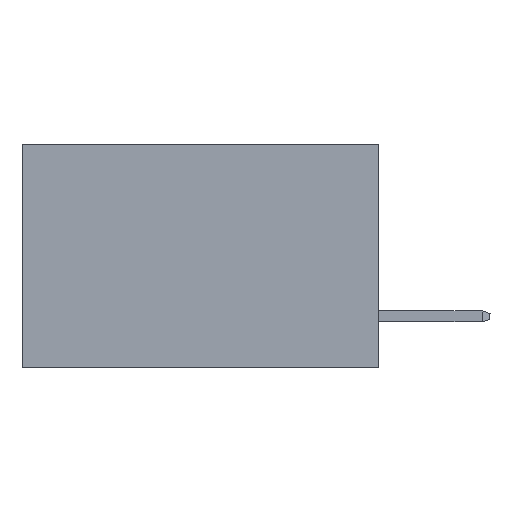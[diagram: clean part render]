
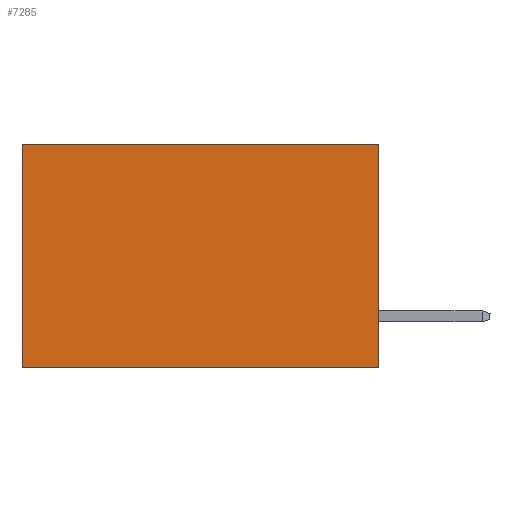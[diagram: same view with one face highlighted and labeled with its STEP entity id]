
A CAD part, left-side view. The second image highlights one B-rep face of the part: STEP entity #7285.
In plain terms, the highlighted planar face has unit normal (-1, 0, 0).
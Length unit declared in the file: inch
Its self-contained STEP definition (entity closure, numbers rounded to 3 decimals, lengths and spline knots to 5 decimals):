
#113 = VERTEX_POINT ( 'NONE', #3536 ) ;
#186 = LINE ( 'NONE', #6970, #7636 ) ;
#222 = CARTESIAN_POINT ( 'NONE',  ( 0.277, 0., -0.37 ) ) ;
#274 = CARTESIAN_POINT ( 'NONE',  ( 0.277, 0., -0.37 ) ) ;
#414 = ORIENTED_EDGE ( 'NONE', *, *, #4793, .F. ) ;
#651 = ORIENTED_EDGE ( 'NONE', *, *, #4095, .F. ) ;
#1653 = VERTEX_POINT ( 'NONE', #2451 ) ;
#1760 = VECTOR ( 'NONE', #8926, 39.37008 ) ;
#1776 = VECTOR ( 'NONE', #3022, 39.37008 ) ;
#1904 = ORIENTED_EDGE ( 'NONE', *, *, #4338, .T. ) ;
#2070 = FACE_OUTER_BOUND ( 'NONE', #3129, .T. ) ;
#2451 = CARTESIAN_POINT ( 'NONE',  ( 0.277, 0.59, 0. ) ) ;
#3022 = DIRECTION ( 'NONE',  ( 0., 0., -1. ) ) ;
#3037 = ORIENTED_EDGE ( 'NONE', *, *, #5791, .T. ) ;
#3129 = EDGE_LOOP ( 'NONE', ( #1904, #414, #651, #3037 ) ) ;
#3536 = CARTESIAN_POINT ( 'NONE',  ( 0.277, 0.59, -0.37 ) ) ;
#3818 = VERTEX_POINT ( 'NONE', #6269 ) ;
#3936 = LINE ( 'NONE', #8883, #1760 ) ;
#4095 = EDGE_CURVE ( 'NONE', #3818, #8555, #186, .T. ) ;
#4338 = EDGE_CURVE ( 'NONE', #1653, #113, #5587, .T. ) ;
#4354 = CARTESIAN_POINT ( 'NONE',  ( 0.277, 0.59, -0.37 ) ) ;
#4793 = EDGE_CURVE ( 'NONE', #8555, #113, #8906, .T. ) ;
#5100 = DIRECTION ( 'NONE',  ( 0., 0., -1. ) ) ;
#5135 = DIRECTION ( 'NONE',  ( 0., 1., 0. ) ) ;
#5587 = LINE ( 'NONE', #4354, #1776 ) ;
#5599 = PLANE ( 'NONE',  #7635 ) ;
#5659 = DIRECTION ( 'NONE',  ( 1., 0., 0. ) ) ;
#5661 = CARTESIAN_POINT ( 'NONE',  ( 0.277, 0., -0.37 ) ) ;
#5791 = EDGE_CURVE ( 'NONE', #3818, #1653, #3936, .T. ) ;
#6269 = CARTESIAN_POINT ( 'NONE',  ( 0.277, 0., 0. ) ) ;
#6970 = CARTESIAN_POINT ( 'NONE',  ( 0.277, 0., -0.37 ) ) ;
#7285 = ADVANCED_FACE ( 'NONE', ( #2070 ), #5599, .F. ) ;
#7377 = DIRECTION ( 'NONE',  ( 0., 0., -1. ) ) ;
#7635 = AXIS2_PLACEMENT_3D ( 'NONE', #5661, #5659, #5100 ) ;
#7636 = VECTOR ( 'NONE', #7377, 39.37008 ) ;
#8555 = VERTEX_POINT ( 'NONE', #274 ) ;
#8684 = VECTOR ( 'NONE', #5135, 39.37008 ) ;
#8883 = CARTESIAN_POINT ( 'NONE',  ( 0.277, 0., 0. ) ) ;
#8906 = LINE ( 'NONE', #222, #8684 ) ;
#8926 = DIRECTION ( 'NONE',  ( 0., 1., 0. ) ) ;
